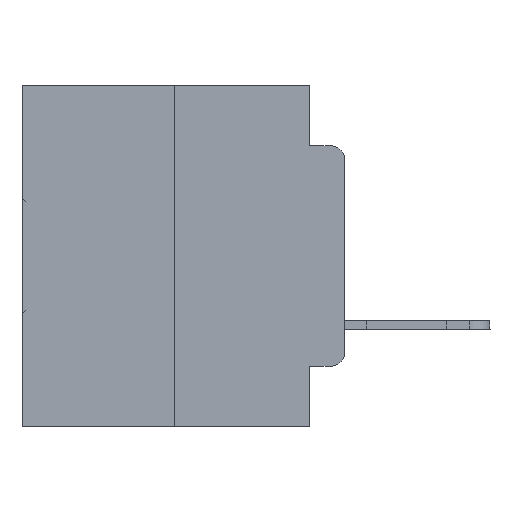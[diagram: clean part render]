
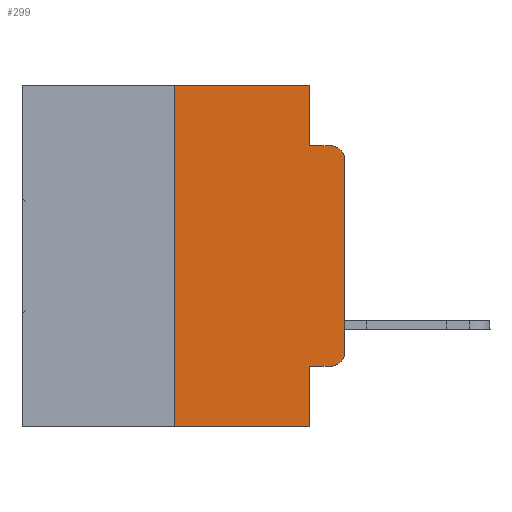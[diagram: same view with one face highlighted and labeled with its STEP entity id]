
A CAD part, left-side view. The second image highlights one B-rep face of the part: STEP entity #299.
In plain terms, the highlighted planar face has unit normal (-1, 0, 0).
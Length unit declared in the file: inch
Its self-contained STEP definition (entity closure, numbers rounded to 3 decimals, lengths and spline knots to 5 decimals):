
#299 = ADVANCED_FACE ( 'NONE', ( #10969 ), #21296, .F. ) ;
#532 = VERTEX_POINT ( 'NONE', #28612 ) ;
#1191 = DIRECTION ( 'NONE',  ( 0., -1., 0. ) ) ;
#1355 = CARTESIAN_POINT ( 'NONE',  ( 0., 0.02, -0.4115 ) ) ;
#1369 = ORIENTED_EDGE ( 'NONE', *, *, #15655, .T. ) ;
#2274 = DIRECTION ( 'NONE',  ( 0., -1., 0. ) ) ;
#2668 = CARTESIAN_POINT ( 'NONE',  ( 0., 0.051, -0.5 ) ) ;
#2782 = LINE ( 'NONE', #29824, #4726 ) ;
#3017 = DIRECTION ( 'NONE',  ( 0., 0., 1. ) ) ;
#3684 = CARTESIAN_POINT ( 'NONE',  ( 0., 0.051, 0. ) ) ;
#4585 = ORIENTED_EDGE ( 'NONE', *, *, #26422, .F. ) ;
#4726 = VECTOR ( 'NONE', #25185, 39.37008 ) ;
#5049 = EDGE_CURVE ( 'NONE', #24613, #532, #6631, .T. ) ;
#5411 = EDGE_CURVE ( 'NONE', #20927, #5976, #20292, .T. ) ;
#5413 = ORIENTED_EDGE ( 'NONE', *, *, #12121, .T. ) ;
#5452 = ORIENTED_EDGE ( 'NONE', *, *, #5411, .F. ) ;
#5609 = VERTEX_POINT ( 'NONE', #14927 ) ;
#5681 = VECTOR ( 'NONE', #21290, 39.37008 ) ;
#5747 = EDGE_CURVE ( 'NONE', #20927, #8064, #13383, .T. ) ;
#5976 = VERTEX_POINT ( 'NONE', #14544 ) ;
#6631 = CIRCLE ( 'NONE', #15263, 0.02 ) ;
#7314 = ORIENTED_EDGE ( 'NONE', *, *, #23844, .F. ) ;
#7425 = EDGE_CURVE ( 'NONE', #16576, #5609, #17078, .T. ) ;
#8064 = VERTEX_POINT ( 'NONE', #2668 ) ;
#8309 = VECTOR ( 'NONE', #28806, 39.37008 ) ;
#9413 = ORIENTED_EDGE ( 'NONE', *, *, #7425, .F. ) ;
#9640 = CARTESIAN_POINT ( 'NONE',  ( 0., 0.473, 0. ) ) ;
#9845 = CARTESIAN_POINT ( 'NONE',  ( 0., 0.25, 0. ) ) ;
#10499 = EDGE_CURVE ( 'NONE', #21764, #18058, #16463, .T. ) ;
#10969 = FACE_OUTER_BOUND ( 'NONE', #20446, .T. ) ;
#11765 = LINE ( 'NONE', #3684, #13639 ) ;
#12121 = EDGE_CURVE ( 'NONE', #18058, #24613, #21697, .T. ) ;
#13383 = LINE ( 'NONE', #25393, #14911 ) ;
#13639 = VECTOR ( 'NONE', #23513, 39.37008 ) ;
#14399 = DIRECTION ( 'NONE',  ( 0., 0., 1. ) ) ;
#14544 = CARTESIAN_POINT ( 'NONE',  ( 0., 0.25, 0. ) ) ;
#14751 = CARTESIAN_POINT ( 'NONE',  ( 0., 0.051, 0. ) ) ;
#14911 = VECTOR ( 'NONE', #1191, 39.37008 ) ;
#14927 = CARTESIAN_POINT ( 'NONE',  ( 0., 0.051, -0.0885 ) ) ;
#15263 = AXIS2_PLACEMENT_3D ( 'NONE', #23175, #25919, #28416 ) ;
#15655 = EDGE_CURVE ( 'NONE', #19064, #21764, #2782, .T. ) ;
#16463 = CIRCLE ( 'NONE', #21114, 0.02 ) ;
#16576 = VERTEX_POINT ( 'NONE', #14751 ) ;
#16931 = CARTESIAN_POINT ( 'NONE',  ( 0., 0.25, -0.5 ) ) ;
#17044 = LINE ( 'NONE', #19266, #8309 ) ;
#17078 = LINE ( 'NONE', #18718, #5681 ) ;
#17251 = CARTESIAN_POINT ( 'NONE',  ( 0., 0.051, -0.4115 ) ) ;
#18058 = VERTEX_POINT ( 'NONE', #31269 ) ;
#18069 = ORIENTED_EDGE ( 'NONE', *, *, #25019, .F. ) ;
#18668 = DIRECTION ( 'NONE',  ( -1., 0., 0. ) ) ;
#18718 = CARTESIAN_POINT ( 'NONE',  ( 0., 0.051, 0. ) ) ;
#19064 = VERTEX_POINT ( 'NONE', #17251 ) ;
#19266 = CARTESIAN_POINT ( 'NONE',  ( 0., 0.051, -0.0885 ) ) ;
#20292 = LINE ( 'NONE', #9845, #21050 ) ;
#20446 = EDGE_LOOP ( 'NONE', ( #5413, #29252, #4585, #9413, #7314, #5452, #30945, #18069, #1369, #23487 ) ) ;
#20927 = VERTEX_POINT ( 'NONE', #16931 ) ;
#21050 = VECTOR ( 'NONE', #14399, 39.37008 ) ;
#21114 = AXIS2_PLACEMENT_3D ( 'NONE', #31103, #18668, #30775 ) ;
#21290 = DIRECTION ( 'NONE',  ( 0., 0., -1. ) ) ;
#21296 = PLANE ( 'NONE',  #30729 ) ;
#21500 = DIRECTION ( 'NONE',  ( 0., 0., -1. ) ) ;
#21697 = LINE ( 'NONE', #24889, #25133 ) ;
#21764 = VERTEX_POINT ( 'NONE', #1355 ) ;
#21771 = VECTOR ( 'NONE', #2274, 39.37008 ) ;
#23175 = CARTESIAN_POINT ( 'NONE',  ( 0., 0.02, -0.1085 ) ) ;
#23487 = ORIENTED_EDGE ( 'NONE', *, *, #10499, .T. ) ;
#23513 = DIRECTION ( 'NONE',  ( 0., 0., -1. ) ) ;
#23844 = EDGE_CURVE ( 'NONE', #5976, #16576, #28295, .T. ) ;
#24613 = VERTEX_POINT ( 'NONE', #27117 ) ;
#24889 = CARTESIAN_POINT ( 'NONE',  ( 0., 0., 0. ) ) ;
#25019 = EDGE_CURVE ( 'NONE', #19064, #8064, #11765, .T. ) ;
#25133 = VECTOR ( 'NONE', #3017, 39.37008 ) ;
#25185 = DIRECTION ( 'NONE',  ( 0., -1., 0. ) ) ;
#25393 = CARTESIAN_POINT ( 'NONE',  ( 0., 0.473, -0.5 ) ) ;
#25919 = DIRECTION ( 'NONE',  ( -1., 0., 0. ) ) ;
#26111 = CARTESIAN_POINT ( 'NONE',  ( 0., 0.473, 0. ) ) ;
#26422 = EDGE_CURVE ( 'NONE', #5609, #532, #17044, .T. ) ;
#27117 = CARTESIAN_POINT ( 'NONE',  ( 0., 0., -0.1085 ) ) ;
#28295 = LINE ( 'NONE', #9640, #21771 ) ;
#28416 = DIRECTION ( 'NONE',  ( 0., 0., -1. ) ) ;
#28612 = CARTESIAN_POINT ( 'NONE',  ( 0., 0.02, -0.0885 ) ) ;
#28806 = DIRECTION ( 'NONE',  ( 0., -1., 0. ) ) ;
#29252 = ORIENTED_EDGE ( 'NONE', *, *, #5049, .T. ) ;
#29824 = CARTESIAN_POINT ( 'NONE',  ( 0., 0.051, -0.4115 ) ) ;
#30729 = AXIS2_PLACEMENT_3D ( 'NONE', #26111, #31278, #21500 ) ;
#30775 = DIRECTION ( 'NONE',  ( 0., 0., -1. ) ) ;
#30945 = ORIENTED_EDGE ( 'NONE', *, *, #5747, .T. ) ;
#31103 = CARTESIAN_POINT ( 'NONE',  ( 0., 0.02, -0.3915 ) ) ;
#31269 = CARTESIAN_POINT ( 'NONE',  ( 0., 0., -0.3915 ) ) ;
#31278 = DIRECTION ( 'NONE',  ( 1., 0., 0. ) ) ;
